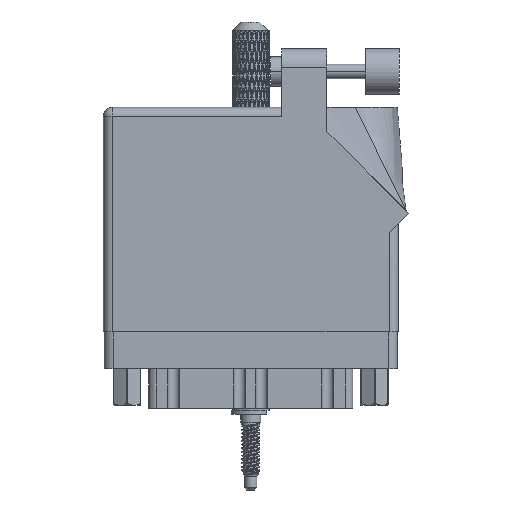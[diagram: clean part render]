
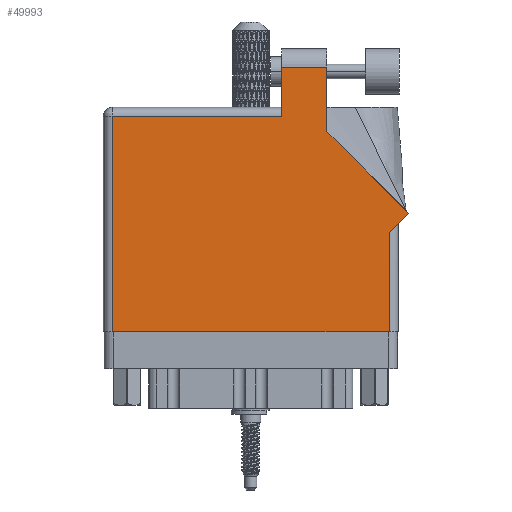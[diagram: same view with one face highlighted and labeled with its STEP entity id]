
A CAD part, front view. The second image highlights one B-rep face of the part: STEP entity #49993.
In plain terms, the highlighted face is planar.
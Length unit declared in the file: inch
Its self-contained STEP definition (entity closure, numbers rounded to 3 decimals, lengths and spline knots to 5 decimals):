
#2318 = VERTEX_POINT ( 'NONE', #29254 ) ;
#2594 = ORIENTED_EDGE ( 'NONE', *, *, #111570, .T. ) ;
#2738 = ORIENTED_EDGE ( 'NONE', *, *, #71956, .T. ) ;
#3400 = VERTEX_POINT ( 'NONE', #4649 ) ;
#4649 = CARTESIAN_POINT ( 'NONE',  ( 1.948, 0., 0. ) ) ;
#6594 = CARTESIAN_POINT ( 'NONE',  ( 0., 1.53, 0. ) ) ;
#7159 = PLANE ( 'NONE',  #69557 ) ;
#8300 = DIRECTION ( 'NONE',  ( 0.707, 0.707, 0. ) ) ;
#9815 = VERTEX_POINT ( 'NONE', #67184 ) ;
#11149 = VECTOR ( 'NONE', #68994, 39.37008 ) ;
#12035 = ORIENTED_EDGE ( 'NONE', *, *, #17662, .T. ) ;
#14475 = LINE ( 'NONE', #73538, #56737 ) ;
#16905 = LINE ( 'NONE', #95444, #21888 ) ;
#17662 = EDGE_CURVE ( 'NONE', #9815, #35181, #16905, .T. ) ;
#19559 = DIRECTION ( 'NONE',  ( -1., 0., 0. ) ) ;
#21413 = CARTESIAN_POINT ( 'NONE',  ( 1.524, 1.36442, 0. ) ) ;
#21520 = VECTOR ( 'NONE', #58766, 39.37008 ) ;
#21645 = ORIENTED_EDGE ( 'NONE', *, *, #98683, .T. ) ;
#21888 = VECTOR ( 'NONE', #8300, 39.37008 ) ;
#22001 = DIRECTION ( 'NONE',  ( 1., 0., 0. ) ) ;
#25479 = ORIENTED_EDGE ( 'NONE', *, *, #77911, .T. ) ;
#26024 = CARTESIAN_POINT ( 'NONE',  ( 0.062, 0., 0. ) ) ;
#27639 = EDGE_CURVE ( 'NONE', #3400, #9815, #109487, .T. ) ;
#28398 = VECTOR ( 'NONE', #56756, 39.37008 ) ;
#29254 = CARTESIAN_POINT ( 'NONE',  ( 1.217, 1.805, 0. ) ) ;
#29311 = CARTESIAN_POINT ( 'NONE',  ( 1.948, 0.737, 0. ) ) ;
#31148 = DIRECTION ( 'NONE',  ( -1., 0., 0. ) ) ;
#31194 = CARTESIAN_POINT ( 'NONE',  ( 0., 0., 0. ) ) ;
#31899 = CARTESIAN_POINT ( 'NONE',  ( 2.08071, 0.80771, 0. ) ) ;
#32100 = DIRECTION ( 'NONE',  ( 0., -1., 0. ) ) ;
#35181 = VERTEX_POINT ( 'NONE', #37585 ) ;
#36338 = LINE ( 'NONE', #70690, #61045 ) ;
#37544 = VERTEX_POINT ( 'NONE', #21413 ) ;
#37585 = CARTESIAN_POINT ( 'NONE',  ( 2.08071, 0.80771, 0. ) ) ;
#38588 = VERTEX_POINT ( 'NONE', #52931 ) ;
#39269 = EDGE_CURVE ( 'NONE', #2318, #38588, #73380, .T. ) ;
#40039 = CARTESIAN_POINT ( 'NONE',  ( 0.062, 1.468, 0. ) ) ;
#45730 = VECTOR ( 'NONE', #32100, 39.37008 ) ;
#46492 = CARTESIAN_POINT ( 'NONE',  ( 0., 1.468, 0. ) ) ;
#48526 = LINE ( 'NONE', #31899, #21520 ) ;
#48730 = EDGE_CURVE ( 'NONE', #104634, #2318, #14475, .T. ) ;
#49993 = ADVANCED_FACE ( 'NONE', ( #75370 ), #7159, .F. ) ;
#52931 = CARTESIAN_POINT ( 'NONE',  ( 1.217, 1.468, 0. ) ) ;
#56737 = VECTOR ( 'NONE', #31148, 39.37008 ) ;
#56756 = DIRECTION ( 'NONE',  ( 0., 1., 0. ) ) ;
#57789 = VERTEX_POINT ( 'NONE', #66063 ) ;
#58766 = DIRECTION ( 'NONE',  ( -0.707, 0.707, 0. ) ) ;
#59669 = VECTOR ( 'NONE', #22001, 39.37008 ) ;
#61045 = VECTOR ( 'NONE', #71249, 39.37008 ) ;
#64766 = ORIENTED_EDGE ( 'NONE', *, *, #27639, .T. ) ;
#66063 = CARTESIAN_POINT ( 'NONE',  ( 0.062, 0., 0. ) ) ;
#67184 = CARTESIAN_POINT ( 'NONE',  ( 1.948, 0.675, 0. ) ) ;
#68994 = DIRECTION ( 'NONE',  ( 0., -1., 0. ) ) ;
#69557 = AXIS2_PLACEMENT_3D ( 'NONE', #6594, #113174, #77636 ) ;
#69742 = VECTOR ( 'NONE', #19559, 39.37008 ) ;
#70690 = CARTESIAN_POINT ( 'NONE',  ( 1.524, 1.36442, 0. ) ) ;
#71249 = DIRECTION ( 'NONE',  ( 0., 1., 0. ) ) ;
#71956 = EDGE_CURVE ( 'NONE', #37544, #104634, #36338, .T. ) ;
#73380 = LINE ( 'NONE', #83688, #45730 ) ;
#73538 = CARTESIAN_POINT ( 'NONE',  ( 1.217, 1.805, 0. ) ) ;
#75370 = FACE_OUTER_BOUND ( 'NONE', #99633, .T. ) ;
#77636 = DIRECTION ( 'NONE',  ( -1., 0., 0. ) ) ;
#77911 = EDGE_CURVE ( 'NONE', #97573, #57789, #94800, .T. ) ;
#81616 = LINE ( 'NONE', #31194, #59669 ) ;
#83688 = CARTESIAN_POINT ( 'NONE',  ( 1.217, 1.53, 0. ) ) ;
#84200 = EDGE_CURVE ( 'NONE', #57789, #3400, #81616, .T. ) ;
#85010 = CARTESIAN_POINT ( 'NONE',  ( 1.524, 1.805, 0. ) ) ;
#94800 = LINE ( 'NONE', #26024, #11149 ) ;
#95444 = CARTESIAN_POINT ( 'NONE',  ( 2.01, 0.737, 0. ) ) ;
#97573 = VERTEX_POINT ( 'NONE', #40039 ) ;
#98683 = EDGE_CURVE ( 'NONE', #35181, #37544, #48526, .T. ) ;
#99633 = EDGE_LOOP ( 'NONE', ( #2738, #105315, #100210, #2594, #25479, #111644, #64766, #12035, #21645 ) ) ;
#100210 = ORIENTED_EDGE ( 'NONE', *, *, #39269, .T. ) ;
#104634 = VERTEX_POINT ( 'NONE', #85010 ) ;
#105315 = ORIENTED_EDGE ( 'NONE', *, *, #48730, .T. ) ;
#107239 = LINE ( 'NONE', #46492, #69742 ) ;
#109487 = LINE ( 'NONE', #29311, #28398 ) ;
#111570 = EDGE_CURVE ( 'NONE', #38588, #97573, #107239, .T. ) ;
#111644 = ORIENTED_EDGE ( 'NONE', *, *, #84200, .T. ) ;
#113174 = DIRECTION ( 'NONE',  ( 0., 0., -1. ) ) ;
